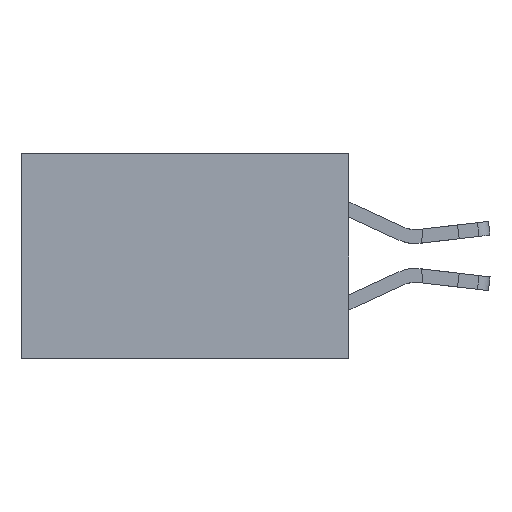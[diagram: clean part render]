
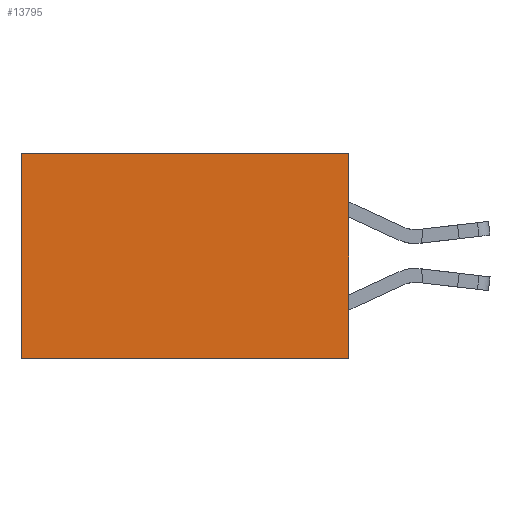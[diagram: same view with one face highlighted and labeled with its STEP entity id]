
A CAD part, left-side view. The second image highlights one B-rep face of the part: STEP entity #13795.
In plain terms, the highlighted planar face has unit normal (-1, 0, 0).
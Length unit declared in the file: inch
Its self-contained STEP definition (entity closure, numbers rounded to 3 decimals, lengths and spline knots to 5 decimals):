
#265 = VERTEX_POINT ( 'NONE', #24514 ) ;
#458 = EDGE_LOOP ( 'NONE', ( #23259, #2891, #17977, #1910 ) ) ;
#1259 = EDGE_CURVE ( 'NONE', #5300, #4716, #18731, .T. ) ;
#1910 = ORIENTED_EDGE ( 'NONE', *, *, #1259, .T. ) ;
#2891 = ORIENTED_EDGE ( 'NONE', *, *, #7565, .F. ) ;
#4506 = CARTESIAN_POINT ( 'NONE',  ( 0.277, 0.59, -0.37 ) ) ;
#4716 = VERTEX_POINT ( 'NONE', #19998 ) ;
#5300 = VERTEX_POINT ( 'NONE', #10898 ) ;
#6382 = CARTESIAN_POINT ( 'NONE',  ( 0.277, 0., -0.37 ) ) ;
#7565 = EDGE_CURVE ( 'NONE', #265, #22532, #15804, .T. ) ;
#9560 = DIRECTION ( 'NONE',  ( 0., 1., 0. ) ) ;
#9766 = VECTOR ( 'NONE', #9560, 39.37008 ) ;
#10235 = PLANE ( 'NONE',  #24799 ) ;
#10666 = EDGE_CURVE ( 'NONE', #5300, #265, #17838, .T. ) ;
#10722 = VECTOR ( 'NONE', #21436, 39.37008 ) ;
#10898 = CARTESIAN_POINT ( 'NONE',  ( 0.277, 0., 0. ) ) ;
#11140 = CARTESIAN_POINT ( 'NONE',  ( 0.277, 0., 0. ) ) ;
#11305 = EDGE_CURVE ( 'NONE', #4716, #22532, #23494, .T. ) ;
#11394 = CARTESIAN_POINT ( 'NONE',  ( 0.277, 0.59, -0.37 ) ) ;
#12135 = DIRECTION ( 'NONE',  ( 0., 0., -1. ) ) ;
#13795 = ADVANCED_FACE ( 'NONE', ( #16814 ), #10235, .F. ) ;
#13825 = CARTESIAN_POINT ( 'NONE',  ( 0.277, 0., -0.37 ) ) ;
#15804 = LINE ( 'NONE', #20473, #10722 ) ;
#15977 = DIRECTION ( 'NONE',  ( 0., 0., -1. ) ) ;
#16814 = FACE_OUTER_BOUND ( 'NONE', #458, .T. ) ;
#17225 = VECTOR ( 'NONE', #19576, 39.37008 ) ;
#17838 = LINE ( 'NONE', #13825, #17225 ) ;
#17977 = ORIENTED_EDGE ( 'NONE', *, *, #10666, .F. ) ;
#18445 = VECTOR ( 'NONE', #15977, 39.37008 ) ;
#18731 = LINE ( 'NONE', #11140, #9766 ) ;
#19576 = DIRECTION ( 'NONE',  ( 0., 0., -1. ) ) ;
#19998 = CARTESIAN_POINT ( 'NONE',  ( 0.277, 0.59, 0. ) ) ;
#20473 = CARTESIAN_POINT ( 'NONE',  ( 0.277, 0., -0.37 ) ) ;
#21436 = DIRECTION ( 'NONE',  ( 0., 1., 0. ) ) ;
#22532 = VERTEX_POINT ( 'NONE', #11394 ) ;
#23259 = ORIENTED_EDGE ( 'NONE', *, *, #11305, .T. ) ;
#23494 = LINE ( 'NONE', #4506, #18445 ) ;
#23557 = DIRECTION ( 'NONE',  ( 1., 0., 0. ) ) ;
#24514 = CARTESIAN_POINT ( 'NONE',  ( 0.277, 0., -0.37 ) ) ;
#24799 = AXIS2_PLACEMENT_3D ( 'NONE', #6382, #23557, #12135 ) ;
